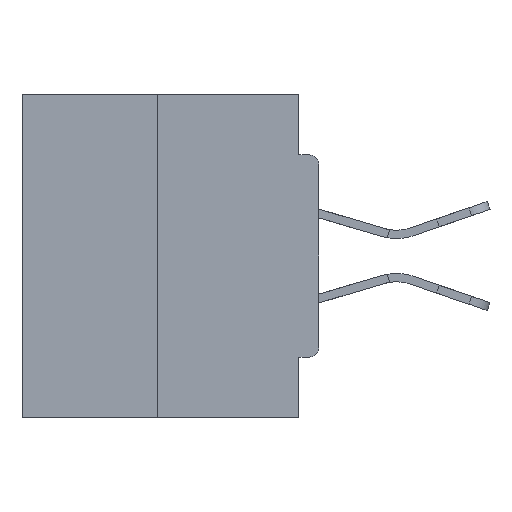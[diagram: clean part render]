
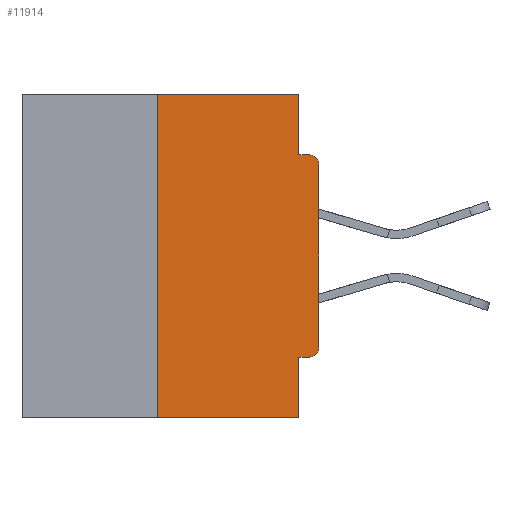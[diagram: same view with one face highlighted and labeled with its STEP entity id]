
A CAD part, left-side view. The second image highlights one B-rep face of the part: STEP entity #11914.
In plain terms, the highlighted planar face has unit normal (-1, 0, 0).
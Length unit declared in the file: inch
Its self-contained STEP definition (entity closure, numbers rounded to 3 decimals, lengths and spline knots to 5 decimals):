
#622 = LINE ( 'NONE', #7734, #6834 ) ;
#933 = DIRECTION ( 'NONE',  ( 0., -1., 0. ) ) ;
#1056 = VECTOR ( 'NONE', #4905, 39.37008 ) ;
#2748 = VECTOR ( 'NONE', #3279, 39.37008 ) ;
#3083 = ORIENTED_EDGE ( 'NONE', *, *, #4951, .T. ) ;
#3279 = DIRECTION ( 'NONE',  ( 0., -1., 0. ) ) ;
#3953 = DIRECTION ( 'NONE',  ( 0., 0., -1. ) ) ;
#4211 = LINE ( 'NONE', #20827, #31506 ) ;
#4265 = CARTESIAN_POINT ( 'NONE',  ( 0., 0., -0.1085 ) ) ;
#4490 = VERTEX_POINT ( 'NONE', #30659 ) ;
#4905 = DIRECTION ( 'NONE',  ( 0., 1., 0. ) ) ;
#4951 = EDGE_CURVE ( 'NONE', #24259, #33758, #19381, .T. ) ;
#5141 = ORIENTED_EDGE ( 'NONE', *, *, #32290, .T. ) ;
#6050 = ORIENTED_EDGE ( 'NONE', *, *, #20720, .F. ) ;
#6255 = VERTEX_POINT ( 'NONE', #19398 ) ;
#6652 = EDGE_CURVE ( 'NONE', #25523, #19793, #4211, .T. ) ;
#6746 = EDGE_CURVE ( 'NONE', #33758, #36453, #622, .T. ) ;
#6834 = VECTOR ( 'NONE', #18600, 39.37008 ) ;
#7131 = CARTESIAN_POINT ( 'NONE',  ( 0., 0.46, -0.5 ) ) ;
#7154 = DIRECTION ( 'NONE',  ( 0., 0., -1. ) ) ;
#7734 = CARTESIAN_POINT ( 'NONE',  ( 0., 0., 0. ) ) ;
#7964 = CARTESIAN_POINT ( 'NONE',  ( 0., 0.015, -0.3915 ) ) ;
#9972 = VERTEX_POINT ( 'NONE', #35957 ) ;
#10545 = CARTESIAN_POINT ( 'NONE',  ( 0., 0.015, -0.0935 ) ) ;
#10652 = VERTEX_POINT ( 'NONE', #27852 ) ;
#11323 = CARTESIAN_POINT ( 'NONE',  ( 0., 0.46, 0. ) ) ;
#11914 = ADVANCED_FACE ( 'NONE', ( #13759 ), #17756, .F. ) ;
#12098 = ORIENTED_EDGE ( 'NONE', *, *, #13598, .T. ) ;
#13247 = AXIS2_PLACEMENT_3D ( 'NONE', #29198, #34822, #3953 ) ;
#13508 = CARTESIAN_POINT ( 'NONE',  ( 0., 0., -0.4065 ) ) ;
#13598 = EDGE_CURVE ( 'NONE', #4490, #10652, #13626, .T. ) ;
#13626 = LINE ( 'NONE', #7131, #32120 ) ;
#13721 = AXIS2_PLACEMENT_3D ( 'NONE', #7964, #36235, #19447 ) ;
#13759 = FACE_OUTER_BOUND ( 'NONE', #15730, .T. ) ;
#14379 = ORIENTED_EDGE ( 'NONE', *, *, #22810, .F. ) ;
#14571 = DIRECTION ( 'NONE',  ( 0., 0., -1. ) ) ;
#15730 = EDGE_LOOP ( 'NONE', ( #14379, #22245, #12098, #19735, #6050, #3083, #26324, #5141, #29177, #30367 ) ) ;
#17756 = PLANE ( 'NONE',  #13247 ) ;
#18469 = CIRCLE ( 'NONE', #33419, 0.015 ) ;
#18600 = DIRECTION ( 'NONE',  ( 0., 0., 1. ) ) ;
#18707 = DIRECTION ( 'NONE',  ( -1., 0., 0. ) ) ;
#19381 = CIRCLE ( 'NONE', #13721, 0.015 ) ;
#19398 = CARTESIAN_POINT ( 'NONE',  ( 0., 0.031, 0. ) ) ;
#19447 = DIRECTION ( 'NONE',  ( 0., 0., -1. ) ) ;
#19735 = ORIENTED_EDGE ( 'NONE', *, *, #33995, .F. ) ;
#19793 = VERTEX_POINT ( 'NONE', #10545 ) ;
#20720 = EDGE_CURVE ( 'NONE', #24259, #9972, #24464, .T. ) ;
#20827 = CARTESIAN_POINT ( 'NONE',  ( 0., 0., -0.0935 ) ) ;
#21175 = LINE ( 'NONE', #21219, #23316 ) ;
#21219 = CARTESIAN_POINT ( 'NONE',  ( 0., 0.031, 0. ) ) ;
#22245 = ORIENTED_EDGE ( 'NONE', *, *, #36426, .F. ) ;
#22810 = EDGE_CURVE ( 'NONE', #34175, #6255, #33590, .T. ) ;
#23316 = VECTOR ( 'NONE', #33004, 39.37008 ) ;
#24259 = VERTEX_POINT ( 'NONE', #32728 ) ;
#24464 = LINE ( 'NONE', #13508, #1056 ) ;
#25012 = LINE ( 'NONE', #29519, #26782 ) ;
#25237 = EDGE_CURVE ( 'NONE', #6255, #25523, #21175, .T. ) ;
#25523 = VERTEX_POINT ( 'NONE', #28324 ) ;
#26324 = ORIENTED_EDGE ( 'NONE', *, *, #6746, .T. ) ;
#26782 = VECTOR ( 'NONE', #29392, 39.37008 ) ;
#27852 = CARTESIAN_POINT ( 'NONE',  ( 0., 0.031, -0.5 ) ) ;
#28027 = CARTESIAN_POINT ( 'NONE',  ( 0., 0.031, -0.5 ) ) ;
#28324 = CARTESIAN_POINT ( 'NONE',  ( 0., 0.031, -0.0935 ) ) ;
#29177 = ORIENTED_EDGE ( 'NONE', *, *, #6652, .F. ) ;
#29198 = CARTESIAN_POINT ( 'NONE',  ( 0., 0.46, 0. ) ) ;
#29392 = DIRECTION ( 'NONE',  ( 0., 0., 1. ) ) ;
#29519 = CARTESIAN_POINT ( 'NONE',  ( 0., 0.25, 0. ) ) ;
#30367 = ORIENTED_EDGE ( 'NONE', *, *, #25237, .F. ) ;
#30392 = CARTESIAN_POINT ( 'NONE',  ( 0., 0., -0.3915 ) ) ;
#30659 = CARTESIAN_POINT ( 'NONE',  ( 0., 0.25, -0.5 ) ) ;
#31506 = VECTOR ( 'NONE', #933, 39.37008 ) ;
#32120 = VECTOR ( 'NONE', #35304, 39.37008 ) ;
#32290 = EDGE_CURVE ( 'NONE', #36453, #19793, #18469, .T. ) ;
#32550 = CARTESIAN_POINT ( 'NONE',  ( 0., 0.25, 0. ) ) ;
#32728 = CARTESIAN_POINT ( 'NONE',  ( 0., 0.015, -0.4065 ) ) ;
#33004 = DIRECTION ( 'NONE',  ( 0., 0., -1. ) ) ;
#33189 = CARTESIAN_POINT ( 'NONE',  ( 0., 0.015, -0.1085 ) ) ;
#33419 = AXIS2_PLACEMENT_3D ( 'NONE', #33189, #18707, #7154 ) ;
#33590 = LINE ( 'NONE', #11323, #2748 ) ;
#33758 = VERTEX_POINT ( 'NONE', #30392 ) ;
#33995 = EDGE_CURVE ( 'NONE', #9972, #10652, #35094, .T. ) ;
#34175 = VERTEX_POINT ( 'NONE', #32550 ) ;
#34822 = DIRECTION ( 'NONE',  ( 1., 0., 0. ) ) ;
#35094 = LINE ( 'NONE', #28027, #35968 ) ;
#35304 = DIRECTION ( 'NONE',  ( 0., -1., 0. ) ) ;
#35957 = CARTESIAN_POINT ( 'NONE',  ( 0., 0.031, -0.4065 ) ) ;
#35968 = VECTOR ( 'NONE', #14571, 39.37008 ) ;
#36235 = DIRECTION ( 'NONE',  ( -1., 0., 0. ) ) ;
#36426 = EDGE_CURVE ( 'NONE', #4490, #34175, #25012, .T. ) ;
#36453 = VERTEX_POINT ( 'NONE', #4265 ) ;
